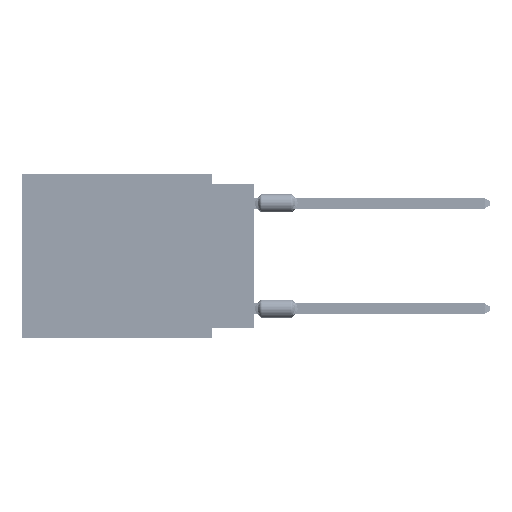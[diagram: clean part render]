
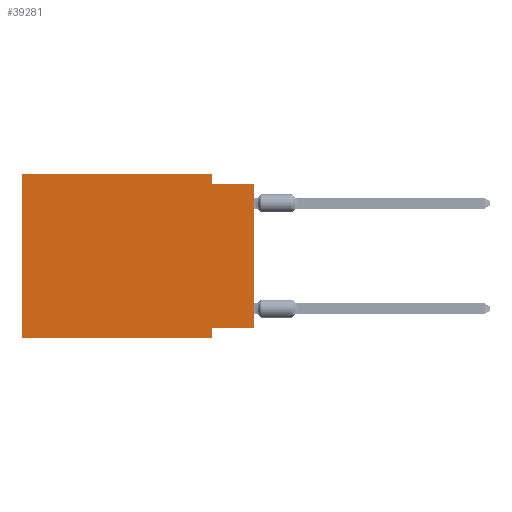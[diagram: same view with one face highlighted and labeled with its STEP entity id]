
A CAD part, left-side view. The second image highlights one B-rep face of the part: STEP entity #39281.
In plain terms, the highlighted planar face has unit normal (-1, 0, 0).
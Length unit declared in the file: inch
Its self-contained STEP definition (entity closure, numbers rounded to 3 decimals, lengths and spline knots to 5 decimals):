
#689 = CARTESIAN_POINT ( 'NONE',  ( 0., 0.55, -0.39 ) ) ;
#729 = AXIS2_PLACEMENT_3D ( 'NONE', #60605, #18717, #6347 ) ;
#2475 = EDGE_CURVE ( 'NONE', #40472, #11327, #36170, .T. ) ;
#2518 = VERTEX_POINT ( 'NONE', #73637 ) ;
#3193 = CARTESIAN_POINT ( 'NONE',  ( 0., 0.1, -0.365 ) ) ;
#4211 = LINE ( 'NONE', #50916, #18233 ) ;
#5144 = CARTESIAN_POINT ( 'NONE',  ( 0., 0.55, 0. ) ) ;
#6347 = DIRECTION ( 'NONE',  ( 0., 0., -1. ) ) ;
#6574 = DIRECTION ( 'NONE',  ( 0., -1., 0. ) ) ;
#7900 = EDGE_CURVE ( 'NONE', #77446, #11327, #36117, .T. ) ;
#9364 = VECTOR ( 'NONE', #11451, 39.37008 ) ;
#11327 = VERTEX_POINT ( 'NONE', #40027 ) ;
#11413 = VERTEX_POINT ( 'NONE', #30324 ) ;
#11451 = DIRECTION ( 'NONE',  ( 0., 0., -1. ) ) ;
#14251 = VECTOR ( 'NONE', #48091, 39.37008 ) ;
#16071 = CARTESIAN_POINT ( 'NONE',  ( 0., 0., -0.025 ) ) ;
#17356 = CARTESIAN_POINT ( 'NONE',  ( 0., 0.55, 0. ) ) ;
#17508 = DIRECTION ( 'NONE',  ( 0., 0., -1. ) ) ;
#17925 = PLANE ( 'NONE',  #729 ) ;
#18151 = CARTESIAN_POINT ( 'NONE',  ( 0., 0.55, -0.39 ) ) ;
#18233 = VECTOR ( 'NONE', #69644, 39.37008 ) ;
#18717 = DIRECTION ( 'NONE',  ( 1., 0., 0. ) ) ;
#19452 = EDGE_CURVE ( 'NONE', #11413, #2518, #48298, .T. ) ;
#21342 = ORIENTED_EDGE ( 'NONE', *, *, #2475, .F. ) ;
#23116 = FACE_OUTER_BOUND ( 'NONE', #45633, .T. ) ;
#23604 = VECTOR ( 'NONE', #6574, 39.37008 ) ;
#23843 = LINE ( 'NONE', #78067, #69146 ) ;
#24040 = EDGE_CURVE ( 'NONE', #40659, #40472, #23843, .T. ) ;
#28977 = ORIENTED_EDGE ( 'NONE', *, *, #59914, .F. ) ;
#30324 = CARTESIAN_POINT ( 'NONE',  ( 0., 0.1, -0.025 ) ) ;
#34413 = EDGE_CURVE ( 'NONE', #43429, #63005, #41718, .T. ) ;
#36117 = LINE ( 'NONE', #18151, #23604 ) ;
#36170 = LINE ( 'NONE', #55320, #9364 ) ;
#39158 = ORIENTED_EDGE ( 'NONE', *, *, #51910, .T. ) ;
#39281 = ADVANCED_FACE ( 'NONE', ( #23116 ), #17925, .F. ) ;
#39320 = VECTOR ( 'NONE', #71820, 39.37008 ) ;
#40027 = CARTESIAN_POINT ( 'NONE',  ( 0., 0.1, -0.39 ) ) ;
#40472 = VERTEX_POINT ( 'NONE', #3193 ) ;
#40659 = VERTEX_POINT ( 'NONE', #48663 ) ;
#40669 = CARTESIAN_POINT ( 'NONE',  ( 0., 0.1, 0. ) ) ;
#41459 = LINE ( 'NONE', #40669, #57477 ) ;
#41540 = LINE ( 'NONE', #52714, #39320 ) ;
#41718 = LINE ( 'NONE', #17356, #14251 ) ;
#43429 = VERTEX_POINT ( 'NONE', #5144 ) ;
#45266 = CARTESIAN_POINT ( 'NONE',  ( 0., 0.1, 0. ) ) ;
#45633 = EDGE_LOOP ( 'NONE', ( #39158, #66116, #52041, #67074, #28977, #64617, #21342, #77124 ) ) ;
#46396 = DIRECTION ( 'NONE',  ( 0., -1., 0. ) ) ;
#48091 = DIRECTION ( 'NONE',  ( 0., -1., 0. ) ) ;
#48298 = LINE ( 'NONE', #16071, #59149 ) ;
#48663 = CARTESIAN_POINT ( 'NONE',  ( 0., 0., -0.365 ) ) ;
#50916 = CARTESIAN_POINT ( 'NONE',  ( 0., 0., 0. ) ) ;
#51910 = EDGE_CURVE ( 'NONE', #40659, #2518, #4211, .T. ) ;
#52041 = ORIENTED_EDGE ( 'NONE', *, *, #61659, .F. ) ;
#52714 = CARTESIAN_POINT ( 'NONE',  ( 0., 0.55, 0. ) ) ;
#55320 = CARTESIAN_POINT ( 'NONE',  ( 0., 0.1, -0.39 ) ) ;
#57477 = VECTOR ( 'NONE', #17508, 39.37008 ) ;
#59149 = VECTOR ( 'NONE', #46396, 39.37008 ) ;
#59914 = EDGE_CURVE ( 'NONE', #77446, #43429, #41540, .T. ) ;
#60605 = CARTESIAN_POINT ( 'NONE',  ( 0., 0.55, 0. ) ) ;
#60935 = DIRECTION ( 'NONE',  ( 0., 1., 0. ) ) ;
#61659 = EDGE_CURVE ( 'NONE', #63005, #11413, #41459, .T. ) ;
#63005 = VERTEX_POINT ( 'NONE', #45266 ) ;
#64617 = ORIENTED_EDGE ( 'NONE', *, *, #7900, .T. ) ;
#66116 = ORIENTED_EDGE ( 'NONE', *, *, #19452, .F. ) ;
#67074 = ORIENTED_EDGE ( 'NONE', *, *, #34413, .F. ) ;
#69146 = VECTOR ( 'NONE', #60935, 39.37008 ) ;
#69644 = DIRECTION ( 'NONE',  ( 0., 0., 1. ) ) ;
#71820 = DIRECTION ( 'NONE',  ( 0., 0., 1. ) ) ;
#73637 = CARTESIAN_POINT ( 'NONE',  ( 0., 0., -0.025 ) ) ;
#77124 = ORIENTED_EDGE ( 'NONE', *, *, #24040, .F. ) ;
#77446 = VERTEX_POINT ( 'NONE', #689 ) ;
#78067 = CARTESIAN_POINT ( 'NONE',  ( 0., 0., -0.365 ) ) ;
